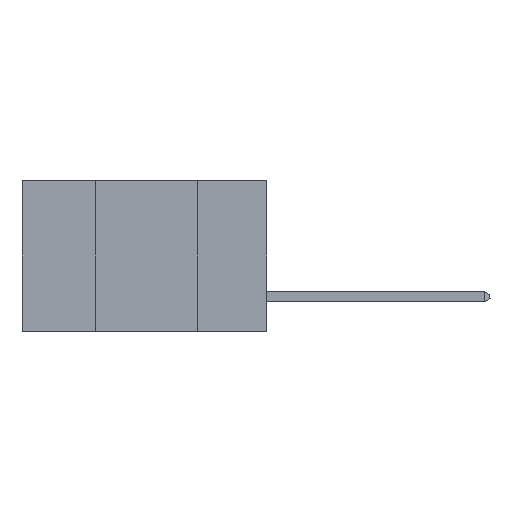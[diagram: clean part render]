
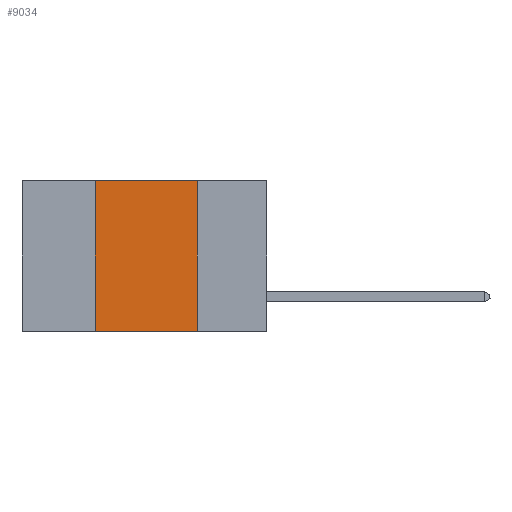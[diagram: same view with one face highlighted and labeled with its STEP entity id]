
A CAD part, left-side view. The second image highlights one B-rep face of the part: STEP entity #9034.
In plain terms, the highlighted planar face has unit normal (-1, 0, 0).
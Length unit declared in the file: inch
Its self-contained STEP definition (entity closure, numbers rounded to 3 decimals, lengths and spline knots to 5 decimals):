
#647 = VECTOR ( 'NONE', #42149, 39.37008 ) ;
#2255 = CARTESIAN_POINT ( 'NONE',  ( 0., 0.6, 0. ) ) ;
#3567 = LINE ( 'NONE', #35587, #35644 ) ;
#6273 = ORIENTED_EDGE ( 'NONE', *, *, #27771, .T. ) ;
#9034 = ADVANCED_FACE ( 'NONE', ( #40025 ), #19740, .F. ) ;
#9297 = CARTESIAN_POINT ( 'NONE',  ( 0., 0.6, 0. ) ) ;
#9384 = VERTEX_POINT ( 'NONE', #32552 ) ;
#10144 = DIRECTION ( 'NONE',  ( 0., 0., 1. ) ) ;
#10422 = VECTOR ( 'NONE', #10144, 39.37008 ) ;
#11461 = DIRECTION ( 'NONE',  ( 0., -1., 0. ) ) ;
#13138 = CARTESIAN_POINT ( 'NONE',  ( 0., 0.42, -0.37 ) ) ;
#13752 = VECTOR ( 'NONE', #11461, 39.37008 ) ;
#14922 = LINE ( 'NONE', #37914, #10422 ) ;
#15662 = VERTEX_POINT ( 'NONE', #13138 ) ;
#15792 = EDGE_CURVE ( 'NONE', #18347, #9384, #3567, .T. ) ;
#18347 = VERTEX_POINT ( 'NONE', #41866 ) ;
#19740 = PLANE ( 'NONE',  #33131 ) ;
#21126 = VERTEX_POINT ( 'NONE', #22140 ) ;
#22140 = CARTESIAN_POINT ( 'NONE',  ( 0., 0.42, 0. ) ) ;
#22666 = LINE ( 'NONE', #9297, #647 ) ;
#23175 = DIRECTION ( 'NONE',  ( 0., 0., -1. ) ) ;
#24500 = EDGE_CURVE ( 'NONE', #15662, #21126, #14922, .T. ) ;
#24648 = CARTESIAN_POINT ( 'NONE',  ( 0., 0.6, -0.37 ) ) ;
#27771 = EDGE_CURVE ( 'NONE', #15662, #9384, #33346, .T. ) ;
#28222 = EDGE_CURVE ( 'NONE', #21126, #18347, #22666, .T. ) ;
#28604 = ORIENTED_EDGE ( 'NONE', *, *, #24500, .F. ) ;
#30000 = ORIENTED_EDGE ( 'NONE', *, *, #28222, .F. ) ;
#31362 = DIRECTION ( 'NONE',  ( 0., 0., -1. ) ) ;
#32552 = CARTESIAN_POINT ( 'NONE',  ( 0., 0.17, -0.37 ) ) ;
#33131 = AXIS2_PLACEMENT_3D ( 'NONE', #2255, #44661, #23175 ) ;
#33346 = LINE ( 'NONE', #24648, #13752 ) ;
#34994 = ORIENTED_EDGE ( 'NONE', *, *, #15792, .F. ) ;
#35587 = CARTESIAN_POINT ( 'NONE',  ( 0., 0.17, 0. ) ) ;
#35644 = VECTOR ( 'NONE', #31362, 39.37008 ) ;
#37914 = CARTESIAN_POINT ( 'NONE',  ( 0., 0.42, 0. ) ) ;
#40025 = FACE_OUTER_BOUND ( 'NONE', #42603, .T. ) ;
#41866 = CARTESIAN_POINT ( 'NONE',  ( 0., 0.17, 0. ) ) ;
#42149 = DIRECTION ( 'NONE',  ( 0., -1., 0. ) ) ;
#42603 = EDGE_LOOP ( 'NONE', ( #34994, #30000, #28604, #6273 ) ) ;
#44661 = DIRECTION ( 'NONE',  ( 1., 0., 0. ) ) ;
